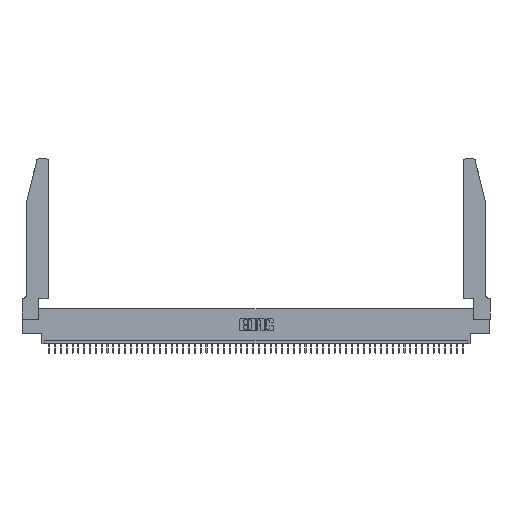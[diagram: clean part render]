
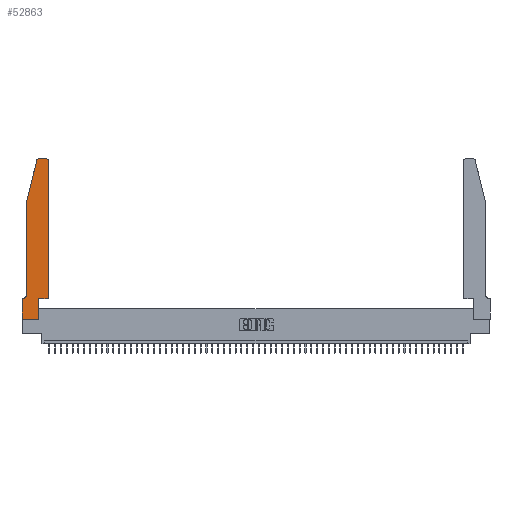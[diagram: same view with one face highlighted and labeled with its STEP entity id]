
A CAD part, top view. The second image highlights one B-rep face of the part: STEP entity #52863.
In plain terms, the highlighted planar face has unit normal (0, 0, 1).
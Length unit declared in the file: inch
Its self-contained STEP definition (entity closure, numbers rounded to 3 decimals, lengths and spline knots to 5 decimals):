
#112 = CARTESIAN_POINT ( 'NONE',  ( 0.0755, 2., 0.37 ) ) ;
#441 = VERTEX_POINT ( 'NONE', #54565 ) ;
#490 = LINE ( 'NONE', #6732, #7764 ) ;
#823 = DIRECTION ( 'NONE',  ( 0., 0., 1. ) ) ;
#932 = DIRECTION ( 'NONE',  ( -1., 0., 0. ) ) ;
#1113 = CARTESIAN_POINT ( 'NONE',  ( 0.284, 2.75, 0.37 ) ) ;
#1249 = CARTESIAN_POINT ( 'NONE',  ( 0.4505, 0.35, 0.37 ) ) ;
#1490 = EDGE_CURVE ( 'NONE', #16182, #19179, #42371, .T. ) ;
#1777 = CARTESIAN_POINT ( 'NONE',  ( 0.4205, 2.72, 0.37 ) ) ;
#2355 = CARTESIAN_POINT ( 'NONE',  ( 0., 0.35, 0.37 ) ) ;
#3163 = VECTOR ( 'NONE', #29319, 39.37008 ) ;
#4761 = CARTESIAN_POINT ( 'NONE',  ( 0.0755, 0.35, 0.37 ) ) ;
#4813 = VERTEX_POINT ( 'NONE', #2355 ) ;
#4981 = EDGE_CURVE ( 'NONE', #441, #41460, #21280, .T. ) ;
#5004 = EDGE_CURVE ( 'NONE', #46810, #4813, #37195, .T. ) ;
#6313 = VERTEX_POINT ( 'NONE', #26363 ) ;
#6531 = EDGE_CURVE ( 'NONE', #19179, #29009, #23109, .T. ) ;
#6596 = VERTEX_POINT ( 'NONE', #27459 ) ;
#6681 = CARTESIAN_POINT ( 'NONE',  ( 0., 0., 0.37 ) ) ;
#6732 = CARTESIAN_POINT ( 'NONE',  ( 0.4505, 0.35, 0.37 ) ) ;
#7308 = VECTOR ( 'NONE', #34632, 39.37008 ) ;
#7764 = VECTOR ( 'NONE', #19730, 39.37008 ) ;
#7959 = CARTESIAN_POINT ( 'NONE',  ( 0.284, 2.72, 0.37 ) ) ;
#8495 = VECTOR ( 'NONE', #31728, 39.37008 ) ;
#8790 = CARTESIAN_POINT ( 'NONE',  ( 0.4505, 2.72, 0.37 ) ) ;
#9310 = DIRECTION ( 'NONE',  ( 0., 0., -1. ) ) ;
#10505 = DIRECTION ( 'NONE',  ( 0., 0., 1. ) ) ;
#10792 = CARTESIAN_POINT ( 'NONE',  ( 0.0755, 2., 0.37 ) ) ;
#12365 = VECTOR ( 'NONE', #16199, 39.37008 ) ;
#12543 = EDGE_CURVE ( 'NONE', #6596, #46810, #44734, .T. ) ;
#12727 = AXIS2_PLACEMENT_3D ( 'NONE', #7959, #37681, #46275 ) ;
#13162 = LINE ( 'NONE', #25377, #35047 ) ;
#13269 = DIRECTION ( 'NONE',  ( 1., 0., 0. ) ) ;
#16182 = VERTEX_POINT ( 'NONE', #6681 ) ;
#16199 = DIRECTION ( 'NONE',  ( -0.239, -0.971, 0. ) ) ;
#16815 = VERTEX_POINT ( 'NONE', #112 ) ;
#17384 = DIRECTION ( 'NONE',  ( -1., 0., 0. ) ) ;
#17401 = ORIENTED_EDGE ( 'NONE', *, *, #5004, .T. ) ;
#17959 = ORIENTED_EDGE ( 'NONE', *, *, #20498, .T. ) ;
#18594 = EDGE_CURVE ( 'NONE', #4813, #16182, #13162, .T. ) ;
#19179 = VERTEX_POINT ( 'NONE', #21039 ) ;
#19460 = EDGE_CURVE ( 'NONE', #6313, #16815, #22337, .T. ) ;
#19730 = DIRECTION ( 'NONE',  ( 1., 0., 0. ) ) ;
#20498 = EDGE_CURVE ( 'NONE', #16815, #6596, #36813, .T. ) ;
#21039 = CARTESIAN_POINT ( 'NONE',  ( 0.2865, 0., 0.37 ) ) ;
#21280 = LINE ( 'NONE', #41921, #45252 ) ;
#21747 = CIRCLE ( 'NONE', #12727, 0.03 ) ;
#22337 = LINE ( 'NONE', #39152, #12365 ) ;
#23109 = LINE ( 'NONE', #27996, #8495 ) ;
#23403 = DIRECTION ( 'NONE',  ( 0., -1., 0. ) ) ;
#23870 = ORIENTED_EDGE ( 'NONE', *, *, #19460, .T. ) ;
#24182 = EDGE_CURVE ( 'NONE', #44832, #441, #31866, .T. ) ;
#24656 = ORIENTED_EDGE ( 'NONE', *, *, #6531, .T. ) ;
#25377 = CARTESIAN_POINT ( 'NONE',  ( 0., 0., 0.37 ) ) ;
#25534 = PLANE ( 'NONE',  #44654 ) ;
#26363 = CARTESIAN_POINT ( 'NONE',  ( 0.25487, 2.72718, 0.37 ) ) ;
#26369 = EDGE_CURVE ( 'NONE', #29009, #41702, #490, .T. ) ;
#27459 = CARTESIAN_POINT ( 'NONE',  ( 0.0755, 0.42, 0.37 ) ) ;
#27996 = CARTESIAN_POINT ( 'NONE',  ( 0.2865, 0.35, 0.37 ) ) ;
#28471 = AXIS2_PLACEMENT_3D ( 'NONE', #47237, #9310, #932 ) ;
#29009 = VERTEX_POINT ( 'NONE', #32426 ) ;
#29210 = AXIS2_PLACEMENT_3D ( 'NONE', #1777, #10505, #48820 ) ;
#29319 = DIRECTION ( 'NONE',  ( 1., 0., 0. ) ) ;
#29663 = DIRECTION ( 'NONE',  ( 0., -1., 0. ) ) ;
#29923 = ORIENTED_EDGE ( 'NONE', *, *, #26369, .T. ) ;
#30954 = ORIENTED_EDGE ( 'NONE', *, *, #46290, .T. ) ;
#31332 = DIRECTION ( 'NONE',  ( 0., 1., 0. ) ) ;
#31728 = DIRECTION ( 'NONE',  ( 0., 1., 0. ) ) ;
#31866 = CIRCLE ( 'NONE', #29210, 0.03 ) ;
#32426 = CARTESIAN_POINT ( 'NONE',  ( 0.2865, 0.35, 0.37 ) ) ;
#33446 = CARTESIAN_POINT ( 'NONE',  ( 0., 0., 0.37 ) ) ;
#34205 = EDGE_LOOP ( 'NONE', ( #50635, #30954, #23870, #17959, #49812, #17401, #42963, #46846, #24656, #29923, #41596, #45264 ) ) ;
#34607 = CARTESIAN_POINT ( 'NONE',  ( 0., 0.35, 0.37 ) ) ;
#34632 = DIRECTION ( 'NONE',  ( -1., 0., 0. ) ) ;
#35047 = VECTOR ( 'NONE', #29663, 39.37008 ) ;
#35692 = LINE ( 'NONE', #1249, #41704 ) ;
#36813 = LINE ( 'NONE', #10792, #50827 ) ;
#37195 = LINE ( 'NONE', #4761, #7308 ) ;
#37681 = DIRECTION ( 'NONE',  ( 0., 0., 1. ) ) ;
#39152 = CARTESIAN_POINT ( 'NONE',  ( 0.0755, 2., 0.37 ) ) ;
#41460 = VERTEX_POINT ( 'NONE', #1113 ) ;
#41596 = ORIENTED_EDGE ( 'NONE', *, *, #49866, .T. ) ;
#41702 = VERTEX_POINT ( 'NONE', #45145 ) ;
#41704 = VECTOR ( 'NONE', #31332, 39.37008 ) ;
#41921 = CARTESIAN_POINT ( 'NONE',  ( 0.2605, 2.75, 0.37 ) ) ;
#42318 = CARTESIAN_POINT ( 'NONE',  ( 0.0055, 0.35, 0.37 ) ) ;
#42371 = LINE ( 'NONE', #33446, #3163 ) ;
#42963 = ORIENTED_EDGE ( 'NONE', *, *, #18594, .T. ) ;
#44654 = AXIS2_PLACEMENT_3D ( 'NONE', #34607, #823, #13269 ) ;
#44734 = CIRCLE ( 'NONE', #28471, 0.07 ) ;
#44832 = VERTEX_POINT ( 'NONE', #8790 ) ;
#45145 = CARTESIAN_POINT ( 'NONE',  ( 0.4505, 0.35, 0.37 ) ) ;
#45252 = VECTOR ( 'NONE', #17384, 39.37008 ) ;
#45264 = ORIENTED_EDGE ( 'NONE', *, *, #24182, .T. ) ;
#46275 = DIRECTION ( 'NONE',  ( 1., 0., 0. ) ) ;
#46290 = EDGE_CURVE ( 'NONE', #41460, #6313, #21747, .T. ) ;
#46810 = VERTEX_POINT ( 'NONE', #42318 ) ;
#46846 = ORIENTED_EDGE ( 'NONE', *, *, #1490, .T. ) ;
#47237 = CARTESIAN_POINT ( 'NONE',  ( 0.0055, 0.42, 0.37 ) ) ;
#48820 = DIRECTION ( 'NONE',  ( 1., 0., 0. ) ) ;
#49812 = ORIENTED_EDGE ( 'NONE', *, *, #12543, .T. ) ;
#49866 = EDGE_CURVE ( 'NONE', #41702, #44832, #35692, .T. ) ;
#50635 = ORIENTED_EDGE ( 'NONE', *, *, #4981, .T. ) ;
#50827 = VECTOR ( 'NONE', #23403, 39.37008 ) ;
#52109 = FACE_OUTER_BOUND ( 'NONE', #34205, .T. ) ;
#52863 = ADVANCED_FACE ( 'NONE', ( #52109 ), #25534, .T. ) ;
#54565 = CARTESIAN_POINT ( 'NONE',  ( 0.4205, 2.75, 0.37 ) ) ;
